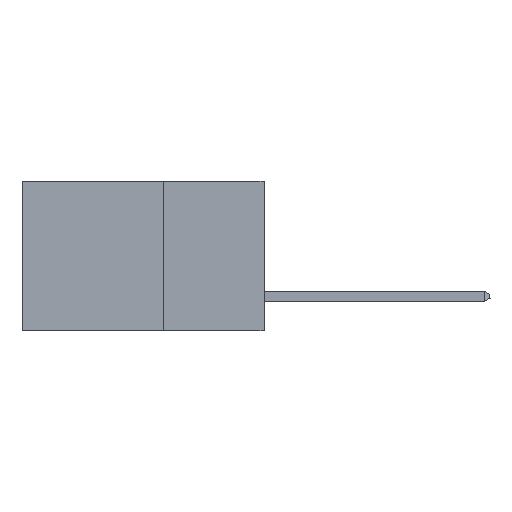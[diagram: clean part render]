
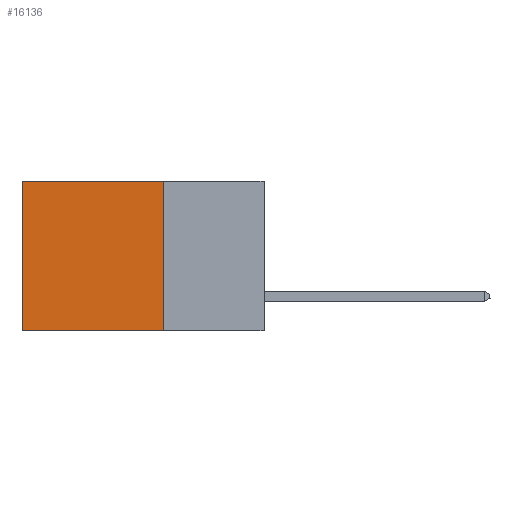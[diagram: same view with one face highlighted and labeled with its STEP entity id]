
A CAD part, left-side view. The second image highlights one B-rep face of the part: STEP entity #16136.
In plain terms, the highlighted planar face has unit normal (-1, 0, 0).
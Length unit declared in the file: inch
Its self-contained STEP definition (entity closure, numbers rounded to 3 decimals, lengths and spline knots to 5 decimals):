
#227 = CARTESIAN_POINT ( 'NONE',  ( 0.298, 0.25, 0. ) ) ;
#249 = CARTESIAN_POINT ( 'NONE',  ( 0.298, 0.25, 0. ) ) ;
#1507 = CARTESIAN_POINT ( 'NONE',  ( 0.298, 0.25, -0.37 ) ) ;
#1982 = CARTESIAN_POINT ( 'NONE',  ( 0.298, 0.6, 0. ) ) ;
#3097 = DIRECTION ( 'NONE',  ( 0., 1., 0. ) ) ;
#3254 = VERTEX_POINT ( 'NONE', #5763 ) ;
#3642 = LINE ( 'NONE', #249, #19683 ) ;
#4659 = EDGE_CURVE ( 'NONE', #5451, #5359, #17127, .T. ) ;
#4681 = VERTEX_POINT ( 'NONE', #1982 ) ;
#5359 = VERTEX_POINT ( 'NONE', #16101 ) ;
#5451 = VERTEX_POINT ( 'NONE', #8562 ) ;
#5728 = CARTESIAN_POINT ( 'NONE',  ( 0.298, 0.6, 0. ) ) ;
#5763 = CARTESIAN_POINT ( 'NONE',  ( 0.298, 0.6, -0.37 ) ) ;
#5798 = DIRECTION ( 'NONE',  ( 0., 0., -1. ) ) ;
#6367 = EDGE_CURVE ( 'NONE', #5359, #3254, #19134, .T. ) ;
#7235 = AXIS2_PLACEMENT_3D ( 'NONE', #227, #14445, #15874 ) ;
#7924 = EDGE_LOOP ( 'NONE', ( #11769, #13973, #10996, #18218 ) ) ;
#8562 = CARTESIAN_POINT ( 'NONE',  ( 0.298, 0.25, 0. ) ) ;
#9574 = PLANE ( 'NONE',  #7235 ) ;
#10095 = EDGE_CURVE ( 'NONE', #4681, #3254, #15294, .T. ) ;
#10996 = ORIENTED_EDGE ( 'NONE', *, *, #4659, .F. ) ;
#11769 = ORIENTED_EDGE ( 'NONE', *, *, #10095, .T. ) ;
#13531 = EDGE_CURVE ( 'NONE', #5451, #4681, #3642, .T. ) ;
#13973 = ORIENTED_EDGE ( 'NONE', *, *, #6367, .F. ) ;
#14197 = DIRECTION ( 'NONE',  ( 0., 1., 0. ) ) ;
#14445 = DIRECTION ( 'NONE',  ( 1., 0., 0. ) ) ;
#14975 = VECTOR ( 'NONE', #3097, 39.37008 ) ;
#15294 = LINE ( 'NONE', #5728, #19203 ) ;
#15874 = DIRECTION ( 'NONE',  ( 0., 0., -1. ) ) ;
#16101 = CARTESIAN_POINT ( 'NONE',  ( 0.298, 0.25, -0.37 ) ) ;
#16136 = ADVANCED_FACE ( 'NONE', ( #17897 ), #9574, .F. ) ;
#17127 = LINE ( 'NONE', #18780, #17610 ) ;
#17610 = VECTOR ( 'NONE', #18717, 39.37008 ) ;
#17897 = FACE_OUTER_BOUND ( 'NONE', #7924, .T. ) ;
#18218 = ORIENTED_EDGE ( 'NONE', *, *, #13531, .T. ) ;
#18717 = DIRECTION ( 'NONE',  ( 0., 0., -1. ) ) ;
#18780 = CARTESIAN_POINT ( 'NONE',  ( 0.298, 0.25, 0. ) ) ;
#19134 = LINE ( 'NONE', #1507, #14975 ) ;
#19203 = VECTOR ( 'NONE', #5798, 39.37008 ) ;
#19683 = VECTOR ( 'NONE', #14197, 39.37008 ) ;
